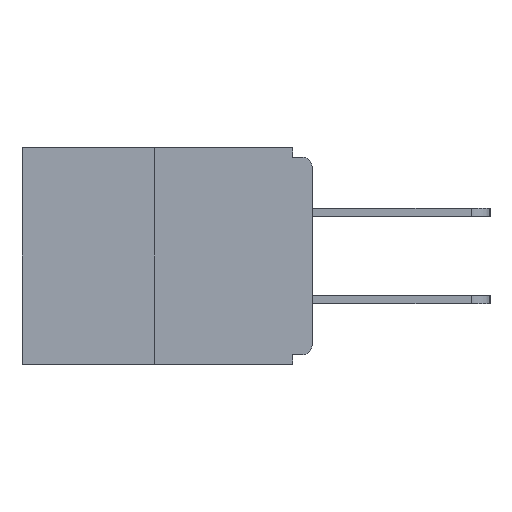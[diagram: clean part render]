
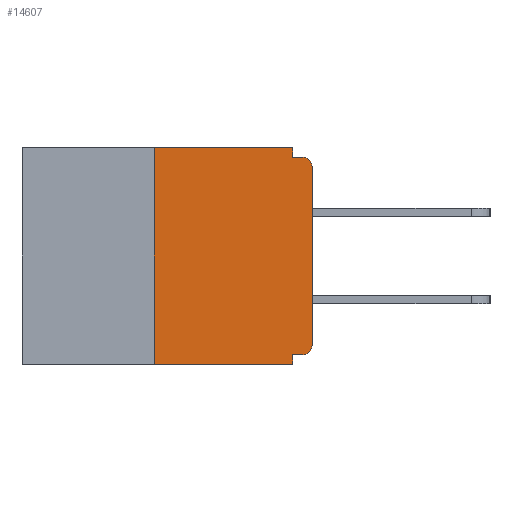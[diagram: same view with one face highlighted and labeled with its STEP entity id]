
A CAD part, left-side view. The second image highlights one B-rep face of the part: STEP entity #14607.
In plain terms, the highlighted planar face has unit normal (-1, 0, 0).
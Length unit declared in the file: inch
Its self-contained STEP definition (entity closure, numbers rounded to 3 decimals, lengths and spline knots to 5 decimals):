
#596 = DIRECTION ( 'NONE',  ( 0., 1., 0. ) ) ;
#763 = DIRECTION ( 'NONE',  ( 0., -1., 0. ) ) ;
#1030 = CIRCLE ( 'NONE', #23259, 0.015 ) ;
#1854 = VERTEX_POINT ( 'NONE', #20882 ) ;
#1889 = EDGE_CURVE ( 'NONE', #28194, #9218, #30163, .T. ) ;
#2238 = AXIS2_PLACEMENT_3D ( 'NONE', #2607, #7254, #26117 ) ;
#2607 = CARTESIAN_POINT ( 'NONE',  ( 0., 0.015, -0.03 ) ) ;
#2787 = VECTOR ( 'NONE', #27834, 39.37008 ) ;
#3777 = VECTOR ( 'NONE', #22010, 39.37008 ) ;
#5244 = EDGE_LOOP ( 'NONE', ( #17421, #30091, #28177, #21749, #8339, #17673, #29918, #21077, #20331, #15609 ) ) ;
#5318 = PLANE ( 'NONE',  #8738 ) ;
#5538 = VECTOR ( 'NONE', #24421, 39.37008 ) ;
#5749 = CARTESIAN_POINT ( 'NONE',  ( 0., 0.46, 0. ) ) ;
#6034 = EDGE_CURVE ( 'NONE', #28727, #18036, #12882, .T. ) ;
#6949 = DIRECTION ( 'NONE',  ( -1., 0., 0. ) ) ;
#7254 = DIRECTION ( 'NONE',  ( -1., 0., 0. ) ) ;
#8339 = ORIENTED_EDGE ( 'NONE', *, *, #29281, .F. ) ;
#8652 = CARTESIAN_POINT ( 'NONE',  ( 0., 0.015, -0.313 ) ) ;
#8738 = AXIS2_PLACEMENT_3D ( 'NONE', #26325, #24481, #19373 ) ;
#8991 = CARTESIAN_POINT ( 'NONE',  ( 0., 0., 0. ) ) ;
#9218 = VERTEX_POINT ( 'NONE', #30274 ) ;
#9958 = FACE_OUTER_BOUND ( 'NONE', #5244, .T. ) ;
#10146 = CIRCLE ( 'NONE', #2238, 0.015 ) ;
#10514 = LINE ( 'NONE', #19925, #17847 ) ;
#10756 = EDGE_CURVE ( 'NONE', #1854, #28194, #1030, .T. ) ;
#11334 = VECTOR ( 'NONE', #28174, 39.37008 ) ;
#11768 = VECTOR ( 'NONE', #22297, 39.37008 ) ;
#12082 = CARTESIAN_POINT ( 'NONE',  ( 0., 0.25, 0. ) ) ;
#12880 = VERTEX_POINT ( 'NONE', #19804 ) ;
#12882 = LINE ( 'NONE', #20594, #21472 ) ;
#13108 = EDGE_CURVE ( 'NONE', #9218, #19095, #10146, .T. ) ;
#14162 = EDGE_CURVE ( 'NONE', #22829, #27712, #24342, .T. ) ;
#14501 = CARTESIAN_POINT ( 'NONE',  ( 0., 0., -0.328 ) ) ;
#14607 = ADVANCED_FACE ( 'NONE', ( #9958 ), #5318, .F. ) ;
#14977 = CARTESIAN_POINT ( 'NONE',  ( 0., 0.46, -0.343 ) ) ;
#15347 = CARTESIAN_POINT ( 'NONE',  ( 0., 0.25, 0. ) ) ;
#15609 = ORIENTED_EDGE ( 'NONE', *, *, #14162, .F. ) ;
#16677 = EDGE_CURVE ( 'NONE', #12880, #18036, #26744, .T. ) ;
#16784 = EDGE_CURVE ( 'NONE', #27712, #19095, #10514, .T. ) ;
#16876 = LINE ( 'NONE', #12082, #11334 ) ;
#17421 = ORIENTED_EDGE ( 'NONE', *, *, #28405, .F. ) ;
#17673 = ORIENTED_EDGE ( 'NONE', *, *, #10756, .T. ) ;
#17847 = VECTOR ( 'NONE', #763, 39.37008 ) ;
#18036 = VERTEX_POINT ( 'NONE', #19965 ) ;
#19095 = VERTEX_POINT ( 'NONE', #20069 ) ;
#19168 = VECTOR ( 'NONE', #596, 39.37008 ) ;
#19373 = DIRECTION ( 'NONE',  ( 0., 0., -1. ) ) ;
#19804 = CARTESIAN_POINT ( 'NONE',  ( 0., 0.25, -0.343 ) ) ;
#19925 = CARTESIAN_POINT ( 'NONE',  ( 0., 0., -0.015 ) ) ;
#19965 = CARTESIAN_POINT ( 'NONE',  ( 0., 0.031, -0.343 ) ) ;
#20069 = CARTESIAN_POINT ( 'NONE',  ( 0., 0.015, -0.015 ) ) ;
#20331 = ORIENTED_EDGE ( 'NONE', *, *, #16784, .F. ) ;
#20594 = CARTESIAN_POINT ( 'NONE',  ( 0., 0.031, -0.343 ) ) ;
#20715 = DIRECTION ( 'NONE',  ( 0., 0., -1. ) ) ;
#20882 = CARTESIAN_POINT ( 'NONE',  ( 0., 0.015, -0.328 ) ) ;
#21077 = ORIENTED_EDGE ( 'NONE', *, *, #13108, .T. ) ;
#21472 = VECTOR ( 'NONE', #27380, 39.37008 ) ;
#21498 = CARTESIAN_POINT ( 'NONE',  ( 0., 0.031, -0.328 ) ) ;
#21749 = ORIENTED_EDGE ( 'NONE', *, *, #6034, .F. ) ;
#22010 = DIRECTION ( 'NONE',  ( 0., 0., -1. ) ) ;
#22297 = DIRECTION ( 'NONE',  ( 0., -1., 0. ) ) ;
#22800 = CARTESIAN_POINT ( 'NONE',  ( 0., 0., -0.313 ) ) ;
#22829 = VERTEX_POINT ( 'NONE', #30278 ) ;
#22981 = CARTESIAN_POINT ( 'NONE',  ( 0., 0.031, -0.015 ) ) ;
#23259 = AXIS2_PLACEMENT_3D ( 'NONE', #8652, #6949, #20715 ) ;
#24034 = VERTEX_POINT ( 'NONE', #15347 ) ;
#24342 = LINE ( 'NONE', #26652, #3777 ) ;
#24421 = DIRECTION ( 'NONE',  ( 0., -1., 0. ) ) ;
#24481 = DIRECTION ( 'NONE',  ( 1., 0., 0. ) ) ;
#26117 = DIRECTION ( 'NONE',  ( 0., 0., -1. ) ) ;
#26255 = LINE ( 'NONE', #14501, #19168 ) ;
#26325 = CARTESIAN_POINT ( 'NONE',  ( 0., 0.46, 0. ) ) ;
#26652 = CARTESIAN_POINT ( 'NONE',  ( 0., 0.031, 0. ) ) ;
#26744 = LINE ( 'NONE', #14977, #5538 ) ;
#26920 = LINE ( 'NONE', #5749, #11768 ) ;
#27380 = DIRECTION ( 'NONE',  ( 0., 0., -1. ) ) ;
#27712 = VERTEX_POINT ( 'NONE', #22981 ) ;
#27834 = DIRECTION ( 'NONE',  ( 0., 0., 1. ) ) ;
#28174 = DIRECTION ( 'NONE',  ( 0., 0., 1. ) ) ;
#28177 = ORIENTED_EDGE ( 'NONE', *, *, #16677, .T. ) ;
#28194 = VERTEX_POINT ( 'NONE', #22800 ) ;
#28405 = EDGE_CURVE ( 'NONE', #24034, #22829, #26920, .T. ) ;
#28727 = VERTEX_POINT ( 'NONE', #21498 ) ;
#29281 = EDGE_CURVE ( 'NONE', #1854, #28727, #26255, .T. ) ;
#29918 = ORIENTED_EDGE ( 'NONE', *, *, #1889, .T. ) ;
#30022 = EDGE_CURVE ( 'NONE', #12880, #24034, #16876, .T. ) ;
#30091 = ORIENTED_EDGE ( 'NONE', *, *, #30022, .F. ) ;
#30163 = LINE ( 'NONE', #8991, #2787 ) ;
#30274 = CARTESIAN_POINT ( 'NONE',  ( 0., 0., -0.03 ) ) ;
#30278 = CARTESIAN_POINT ( 'NONE',  ( 0., 0.031, 0. ) ) ;
